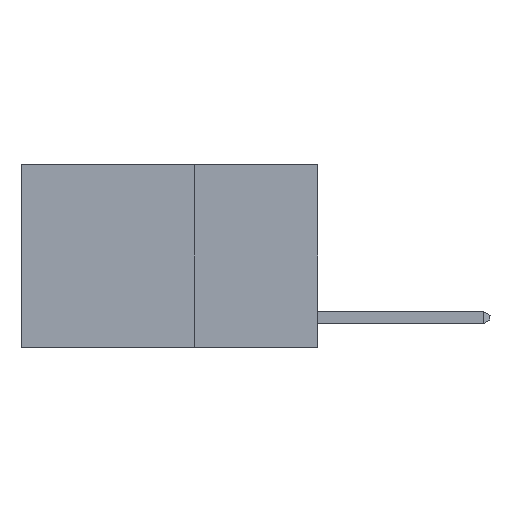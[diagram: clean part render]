
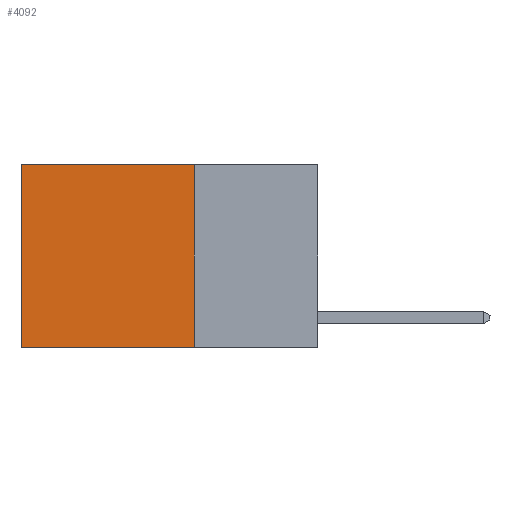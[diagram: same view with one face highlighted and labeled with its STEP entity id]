
A CAD part, left-side view. The second image highlights one B-rep face of the part: STEP entity #4092.
In plain terms, the highlighted planar face has unit normal (-1, 0, 0).
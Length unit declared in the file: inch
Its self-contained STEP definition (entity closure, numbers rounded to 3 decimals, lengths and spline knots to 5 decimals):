
#172 = EDGE_CURVE ( 'NONE', #1114, #6415, #11578, .T. ) ;
#239 = DIRECTION ( 'NONE',  ( 0., 0., -1. ) ) ;
#411 = DIRECTION ( 'NONE',  ( 0., 1., 0. ) ) ;
#515 = DIRECTION ( 'NONE',  ( 0., 0., -1. ) ) ;
#642 = EDGE_CURVE ( 'NONE', #4355, #6415, #11561, .T. ) ;
#865 = EDGE_LOOP ( 'NONE', ( #1148, #4250, #2107, #5355 ) ) ;
#1114 = VERTEX_POINT ( 'NONE', #3989 ) ;
#1148 = ORIENTED_EDGE ( 'NONE', *, *, #172, .T. ) ;
#1449 = CARTESIAN_POINT ( 'NONE',  ( 0.2625, 0.25, 0. ) ) ;
#1742 = CARTESIAN_POINT ( 'NONE',  ( 0.2625, 0.25, -0.37 ) ) ;
#1821 = EDGE_CURVE ( 'NONE', #13039, #1114, #9116, .T. ) ;
#2107 = ORIENTED_EDGE ( 'NONE', *, *, #12662, .F. ) ;
#3989 = CARTESIAN_POINT ( 'NONE',  ( 0.2625, 0.6, 0. ) ) ;
#4092 = ADVANCED_FACE ( 'NONE', ( #9311 ), #13706, .F. ) ;
#4250 = ORIENTED_EDGE ( 'NONE', *, *, #642, .F. ) ;
#4355 = VERTEX_POINT ( 'NONE', #10885 ) ;
#4865 = AXIS2_PLACEMENT_3D ( 'NONE', #12564, #12629, #515 ) ;
#5355 = ORIENTED_EDGE ( 'NONE', *, *, #1821, .T. ) ;
#6101 = DIRECTION ( 'NONE',  ( 0., 1., 0. ) ) ;
#6415 = VERTEX_POINT ( 'NONE', #8420 ) ;
#6909 = CARTESIAN_POINT ( 'NONE',  ( 0.2625, 0.25, 0. ) ) ;
#7585 = VECTOR ( 'NONE', #10642, 39.37008 ) ;
#8420 = CARTESIAN_POINT ( 'NONE',  ( 0.2625, 0.6, -0.37 ) ) ;
#8751 = VECTOR ( 'NONE', #239, 39.37008 ) ;
#9063 = VECTOR ( 'NONE', #411, 39.37008 ) ;
#9116 = LINE ( 'NONE', #12511, #9063 ) ;
#9311 = FACE_OUTER_BOUND ( 'NONE', #865, .T. ) ;
#10642 = DIRECTION ( 'NONE',  ( 0., 0., -1. ) ) ;
#10885 = CARTESIAN_POINT ( 'NONE',  ( 0.2625, 0.25, -0.37 ) ) ;
#10954 = VECTOR ( 'NONE', #6101, 39.37008 ) ;
#11192 = LINE ( 'NONE', #1449, #8751 ) ;
#11561 = LINE ( 'NONE', #1742, #10954 ) ;
#11578 = LINE ( 'NONE', #13735, #7585 ) ;
#12511 = CARTESIAN_POINT ( 'NONE',  ( 0.2625, 0.25, 0. ) ) ;
#12564 = CARTESIAN_POINT ( 'NONE',  ( 0.2625, 0.25, 0. ) ) ;
#12629 = DIRECTION ( 'NONE',  ( 1., 0., 0. ) ) ;
#12662 = EDGE_CURVE ( 'NONE', #13039, #4355, #11192, .T. ) ;
#13039 = VERTEX_POINT ( 'NONE', #6909 ) ;
#13706 = PLANE ( 'NONE',  #4865 ) ;
#13735 = CARTESIAN_POINT ( 'NONE',  ( 0.2625, 0.6, 0. ) ) ;
